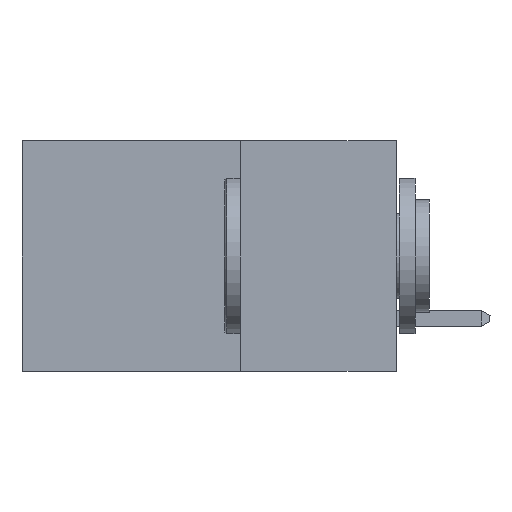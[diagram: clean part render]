
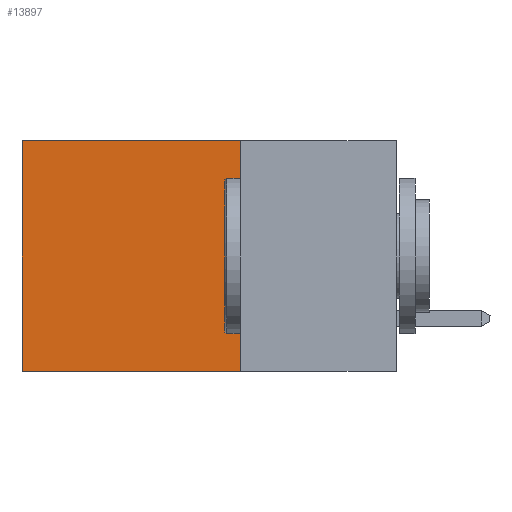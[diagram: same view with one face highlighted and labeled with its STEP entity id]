
A CAD part, left-side view. The second image highlights one B-rep face of the part: STEP entity #13897.
In plain terms, the highlighted planar face has unit normal (-1, 0, 0).
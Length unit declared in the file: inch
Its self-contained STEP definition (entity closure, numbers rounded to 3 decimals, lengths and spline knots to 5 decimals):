
#45 = CARTESIAN_POINT ( 'NONE',  ( 0.2615, 0.6, -0.37 ) ) ;
#1248 = VECTOR ( 'NONE', #15449, 39.37008 ) ;
#2005 = CARTESIAN_POINT ( 'NONE',  ( 0.2615, 0.25, 0. ) ) ;
#2092 = VERTEX_POINT ( 'NONE', #11385 ) ;
#2698 = LINE ( 'NONE', #23339, #18106 ) ;
#3816 = PLANE ( 'NONE',  #11825 ) ;
#4301 = CARTESIAN_POINT ( 'NONE',  ( 0.2615, 0.25, -0.37 ) ) ;
#4337 = VERTEX_POINT ( 'NONE', #2005 ) ;
#5738 = VECTOR ( 'NONE', #24356, 39.37008 ) ;
#5798 = DIRECTION ( 'NONE',  ( 1., 0., 0. ) ) ;
#6383 = LINE ( 'NONE', #4301, #5738 ) ;
#7010 = ORIENTED_EDGE ( 'NONE', *, *, #15974, .T. ) ;
#7974 = VERTEX_POINT ( 'NONE', #20055 ) ;
#8549 = VERTEX_POINT ( 'NONE', #45 ) ;
#10979 = CARTESIAN_POINT ( 'NONE',  ( 0.2615, 0.25, -0.37 ) ) ;
#11005 = FACE_OUTER_BOUND ( 'NONE', #16596, .T. ) ;
#11385 = CARTESIAN_POINT ( 'NONE',  ( 0.2615, 0.6, 0. ) ) ;
#11752 = ORIENTED_EDGE ( 'NONE', *, *, #19170, .F. ) ;
#11825 = AXIS2_PLACEMENT_3D ( 'NONE', #23711, #5798, #19911 ) ;
#13419 = CARTESIAN_POINT ( 'NONE',  ( 0.2615, 0.25, 0. ) ) ;
#13774 = VECTOR ( 'NONE', #22943, 39.37008 ) ;
#13897 = ADVANCED_FACE ( 'NONE', ( #11005 ), #3816, .F. ) ;
#15449 = DIRECTION ( 'NONE',  ( 0., 1., 0. ) ) ;
#15903 = ORIENTED_EDGE ( 'NONE', *, *, #21210, .F. ) ;
#15974 = EDGE_CURVE ( 'NONE', #2092, #8549, #2698, .T. ) ;
#16596 = EDGE_LOOP ( 'NONE', ( #7010, #15903, #11752, #25617 ) ) ;
#17352 = DIRECTION ( 'NONE',  ( 0., 0., -1. ) ) ;
#17913 = LINE ( 'NONE', #13419, #1248 ) ;
#17974 = EDGE_CURVE ( 'NONE', #4337, #2092, #17913, .T. ) ;
#18106 = VECTOR ( 'NONE', #17352, 39.37008 ) ;
#19170 = EDGE_CURVE ( 'NONE', #4337, #7974, #25575, .T. ) ;
#19911 = DIRECTION ( 'NONE',  ( 0., 0., -1. ) ) ;
#20055 = CARTESIAN_POINT ( 'NONE',  ( 0.2615, 0.25, -0.37 ) ) ;
#21210 = EDGE_CURVE ( 'NONE', #7974, #8549, #6383, .T. ) ;
#22943 = DIRECTION ( 'NONE',  ( 0., 0., -1. ) ) ;
#23339 = CARTESIAN_POINT ( 'NONE',  ( 0.2615, 0.6, -0.37 ) ) ;
#23711 = CARTESIAN_POINT ( 'NONE',  ( 0.2615, 0.25, -0.37 ) ) ;
#24356 = DIRECTION ( 'NONE',  ( 0., 1., 0. ) ) ;
#25575 = LINE ( 'NONE', #10979, #13774 ) ;
#25617 = ORIENTED_EDGE ( 'NONE', *, *, #17974, .T. ) ;
